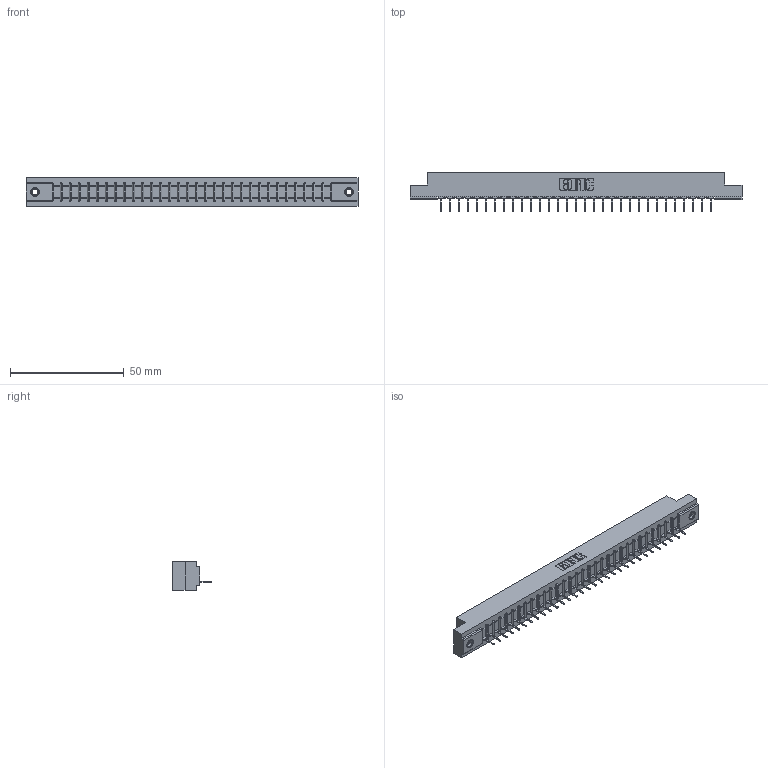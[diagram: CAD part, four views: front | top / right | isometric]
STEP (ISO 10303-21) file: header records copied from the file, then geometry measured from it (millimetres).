
FILE_DESCRIPTION (( 'STEP AP203' ), '1' );
FILE_NAME ('307-031-531-107.STEP', '2019-09-04T00:36:13', ( '' ), ( '' ), 'SwSTEP 2.0', 'SolidWorks 2016', '' );
FILE_SCHEMA (( 'CONFIG_CONTROL_DESIGN' ));
Length unit declared in the file: inch
Products named in the file (4): 345-250-001_345-250-005-103; 307-290-001_531; 307-031-531-107; 307 Part_.156 Dia Mounting Holes
Assembly tree (34 placements, depth 2):
  307-031-531-107
    307 Part_.156 Dia Mounting Holes
    307-290-001_531  x31
    345-250-001_345-250-005-103  x2
Bounding box: 145.85 x 17.42 x 12.7 mm (x, y, z)
Volume: 15007.6 mm3; surface area: 15442.4 mm2
Topology: 34 solids, 34 shells, 1946 faces, 5481 edges, 3518 vertices
Faces by surface type: plane 1249, cylinder 617, sphere 64, cone 12, torus 4
Entity records: 29085 total; most frequent: CARTESIAN_POINT 4875, ORIENTED_EDGE 4854, DIRECTION 4757, EDGE_CURVE 2427, VECTOR 1857, LINE 1857, VERTEX_POINT 1568, AXIS2_PLACEMENT_3D 1450
